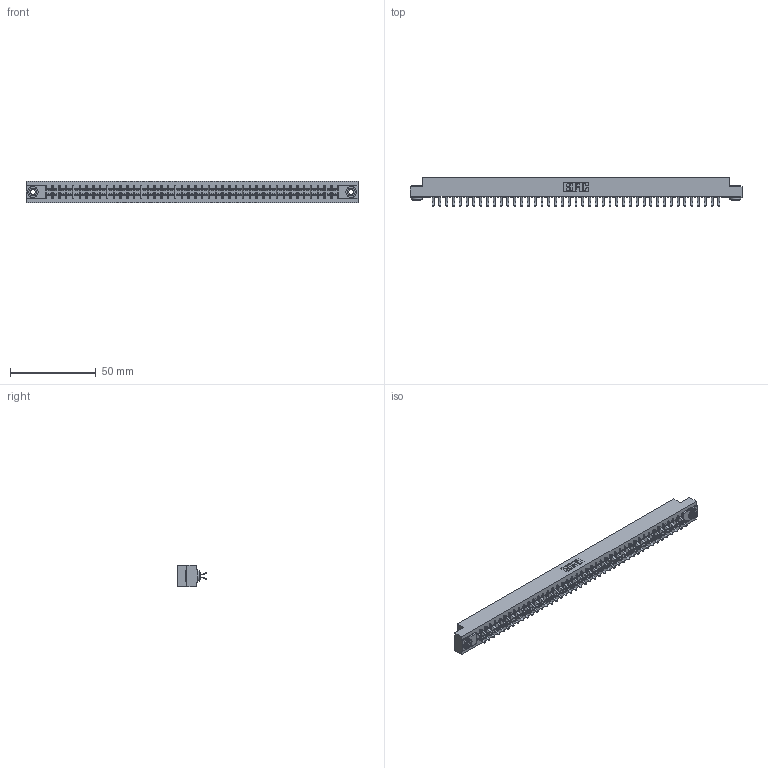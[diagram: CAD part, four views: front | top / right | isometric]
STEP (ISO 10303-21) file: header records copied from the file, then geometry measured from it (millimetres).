
FILE_DESCRIPTION (( 'STEP AP203' ), '1' );
FILE_NAME ('355-086-556-503.STEP', '2019-09-13T17:05:31', ( '' ), ( '' ), 'SwSTEP 2.0', 'SolidWorks 2016', '' );
FILE_SCHEMA (( 'CONFIG_CONTROL_DESIGN' ));
Length unit declared in the file: inch
Products named in the file (4): 305-290-001_556; 345-250-002_345-250-002-102; 355-086-556-503; 305 Part_.156 Dia
Assembly tree (89 placements, depth 2):
  355-086-556-503
    305 Part_.156 Dia
    305-290-001_556  x86
    345-250-002_345-250-002-102  x2
Bounding box: 193.4 x 16.64 x 12.7 mm (x, y, z)
Volume: 19576.3 mm3; surface area: 26157.5 mm2
Topology: 89 solids, 89 shells, 4984 faces, 14317 edges, 9310 vertices
Faces by surface type: plane 2758, cylinder 2046, sphere 172, cone 8
Entity records: 47723 total; most frequent: CARTESIAN_POINT 7880, ORIENTED_EDGE 7814, DIRECTION 7641, EDGE_CURVE 3907, LINE 3147, VECTOR 3147, VERTEX_POINT 2486, AXIS2_PLACEMENT_3D 2247
